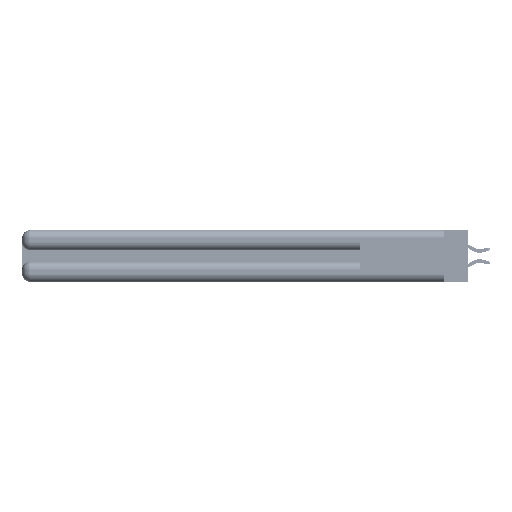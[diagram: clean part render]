
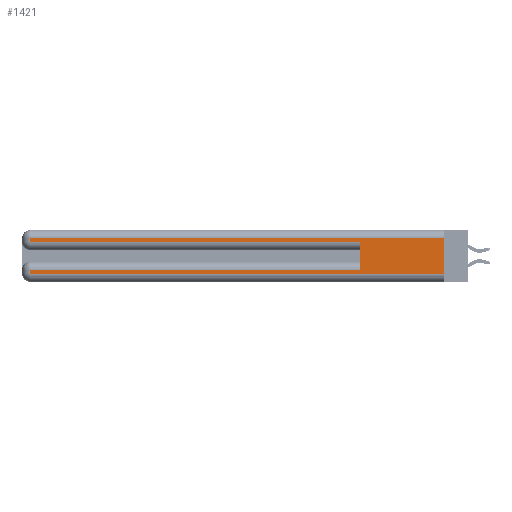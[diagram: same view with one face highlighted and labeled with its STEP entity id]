
A CAD part, left-side view. The second image highlights one B-rep face of the part: STEP entity #1421.
In plain terms, the highlighted planar face has unit normal (-1, 0, 0).
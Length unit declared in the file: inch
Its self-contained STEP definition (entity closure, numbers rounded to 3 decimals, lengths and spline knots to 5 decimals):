
#823 = VECTOR ( 'NONE', #41772, 39.37008 ) ;
#1115 = VECTOR ( 'NONE', #25066, 39.37008 ) ;
#1421 = ADVANCED_FACE ( 'NONE', ( #2305 ), #3438, .F. ) ;
#2055 = LINE ( 'NONE', #49179, #44186 ) ;
#2305 = FACE_OUTER_BOUND ( 'NONE', #45666, .T. ) ;
#3438 = PLANE ( 'NONE',  #17352 ) ;
#4357 = EDGE_CURVE ( 'NONE', #21525, #29761, #2055, .T. ) ;
#4623 = VECTOR ( 'NONE', #31997, 39.37008 ) ;
#7359 = CARTESIAN_POINT ( 'NONE',  ( 0., 0., 0.085 ) ) ;
#7551 = DIRECTION ( 'NONE',  ( 1., 0., 0. ) ) ;
#7585 = CARTESIAN_POINT ( 'NONE',  ( 0., 2.94, 0.37 ) ) ;
#9015 = LINE ( 'NONE', #43099, #29471 ) ;
#10271 = VERTEX_POINT ( 'NONE', #20192 ) ;
#10279 = CARTESIAN_POINT ( 'NONE',  ( 0., 0.6, 0.145 ) ) ;
#10561 = VERTEX_POINT ( 'NONE', #18036 ) ;
#11486 = DIRECTION ( 'NONE',  ( 0., 1., 0. ) ) ;
#12670 = DIRECTION ( 'NONE',  ( 0., 0., -1. ) ) ;
#15539 = CARTESIAN_POINT ( 'NONE',  ( 0., 2.94, 0.31 ) ) ;
#15828 = DIRECTION ( 'NONE',  ( 0., 0., -1. ) ) ;
#16159 = ORIENTED_EDGE ( 'NONE', *, *, #4357, .F. ) ;
#16312 = CARTESIAN_POINT ( 'NONE',  ( 0., 0., 0.31 ) ) ;
#17352 = AXIS2_PLACEMENT_3D ( 'NONE', #32016, #7551, #36128 ) ;
#17597 = EDGE_CURVE ( 'NONE', #22043, #10561, #22744, .T. ) ;
#18036 = CARTESIAN_POINT ( 'NONE',  ( 0., 2.94, 0.285 ) ) ;
#18431 = ORIENTED_EDGE ( 'NONE', *, *, #43204, .T. ) ;
#19766 = ORIENTED_EDGE ( 'NONE', *, *, #48912, .T. ) ;
#20192 = CARTESIAN_POINT ( 'NONE',  ( 0., 2.94, 0.085 ) ) ;
#20435 = CARTESIAN_POINT ( 'NONE',  ( 0., 0., 0.06 ) ) ;
#21525 = VERTEX_POINT ( 'NONE', #16312 ) ;
#22043 = VERTEX_POINT ( 'NONE', #15539 ) ;
#22744 = LINE ( 'NONE', #7585, #33608 ) ;
#23812 = CARTESIAN_POINT ( 'NONE',  ( 0., 0.6, 0.085 ) ) ;
#25066 = DIRECTION ( 'NONE',  ( 0., 0., -1. ) ) ;
#26216 = ORIENTED_EDGE ( 'NONE', *, *, #29497, .F. ) ;
#26246 = CARTESIAN_POINT ( 'NONE',  ( 0., 0., 0.31 ) ) ;
#26396 = LINE ( 'NONE', #27895, #4623 ) ;
#26702 = ORIENTED_EDGE ( 'NONE', *, *, #17597, .T. ) ;
#27895 = CARTESIAN_POINT ( 'NONE',  ( 0., 0., 0.285 ) ) ;
#29303 = LINE ( 'NONE', #10279, #49693 ) ;
#29471 = VECTOR ( 'NONE', #47186, 39.37008 ) ;
#29497 = EDGE_CURVE ( 'NONE', #49100, #49548, #29303, .T. ) ;
#29761 = VERTEX_POINT ( 'NONE', #20435 ) ;
#29829 = LINE ( 'NONE', #7359, #50202 ) ;
#30198 = ORIENTED_EDGE ( 'NONE', *, *, #32735, .T. ) ;
#31997 = DIRECTION ( 'NONE',  ( 0., -1., 0. ) ) ;
#32016 = CARTESIAN_POINT ( 'NONE',  ( 0., 0., 0.37 ) ) ;
#32735 = EDGE_CURVE ( 'NONE', #10561, #49548, #26396, .T. ) ;
#33388 = LINE ( 'NONE', #26246, #823 ) ;
#33608 = VECTOR ( 'NONE', #15828, 39.37008 ) ;
#36128 = DIRECTION ( 'NONE',  ( 0., 0., -1. ) ) ;
#36272 = CARTESIAN_POINT ( 'NONE',  ( 0., 0.6, 0.285 ) ) ;
#36511 = EDGE_CURVE ( 'NONE', #10271, #41047, #52792, .T. ) ;
#41047 = VERTEX_POINT ( 'NONE', #51359 ) ;
#41772 = DIRECTION ( 'NONE',  ( 0., 1., 0. ) ) ;
#42921 = DIRECTION ( 'NONE',  ( 0., 0., 1. ) ) ;
#43099 = CARTESIAN_POINT ( 'NONE',  ( 0., 0., 0.06 ) ) ;
#43204 = EDGE_CURVE ( 'NONE', #49100, #10271, #29829, .T. ) ;
#44186 = VECTOR ( 'NONE', #12670, 39.37008 ) ;
#45387 = CARTESIAN_POINT ( 'NONE',  ( 0., 2.94, 0.37 ) ) ;
#45513 = ORIENTED_EDGE ( 'NONE', *, *, #46157, .T. ) ;
#45666 = EDGE_LOOP ( 'NONE', ( #16159, #45513, #26702, #30198, #26216, #18431, #52471, #19766 ) ) ;
#46157 = EDGE_CURVE ( 'NONE', #21525, #22043, #33388, .T. ) ;
#47186 = DIRECTION ( 'NONE',  ( 0., -1., 0. ) ) ;
#48912 = EDGE_CURVE ( 'NONE', #41047, #29761, #9015, .T. ) ;
#49100 = VERTEX_POINT ( 'NONE', #23812 ) ;
#49179 = CARTESIAN_POINT ( 'NONE',  ( 0., 0., 0.37 ) ) ;
#49548 = VERTEX_POINT ( 'NONE', #36272 ) ;
#49693 = VECTOR ( 'NONE', #42921, 39.37008 ) ;
#50202 = VECTOR ( 'NONE', #11486, 39.37008 ) ;
#51359 = CARTESIAN_POINT ( 'NONE',  ( 0., 2.94, 0.06 ) ) ;
#52471 = ORIENTED_EDGE ( 'NONE', *, *, #36511, .T. ) ;
#52792 = LINE ( 'NONE', #45387, #1115 ) ;
